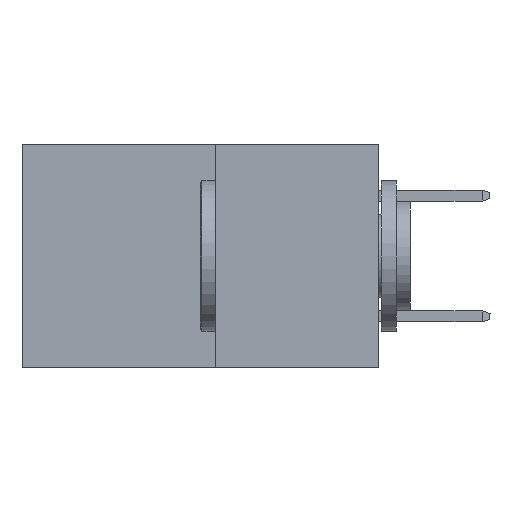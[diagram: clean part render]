
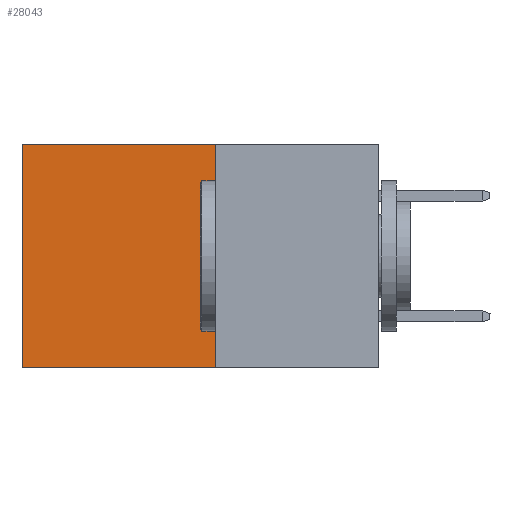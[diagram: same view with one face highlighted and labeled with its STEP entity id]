
A CAD part, left-side view. The second image highlights one B-rep face of the part: STEP entity #28043.
In plain terms, the highlighted planar face has unit normal (-1, 0, 0).
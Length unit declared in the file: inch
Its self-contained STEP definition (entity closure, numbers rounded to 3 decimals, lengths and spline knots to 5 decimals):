
#4459 = LINE ( 'NONE', #9583, #25312 ) ;
#6172 = CARTESIAN_POINT ( 'NONE',  ( 0.277, 0.27, -0.37 ) ) ;
#7576 = VERTEX_POINT ( 'NONE', #14324 ) ;
#8470 = CARTESIAN_POINT ( 'NONE',  ( 0.277, 0.27, -0.37 ) ) ;
#8761 = VECTOR ( 'NONE', #29375, 39.37008 ) ;
#8763 = LINE ( 'NONE', #15173, #21010 ) ;
#8813 = DIRECTION ( 'NONE',  ( 0., 0., -1. ) ) ;
#9583 = CARTESIAN_POINT ( 'NONE',  ( 0.277, 0.59, -0.37 ) ) ;
#9829 = CARTESIAN_POINT ( 'NONE',  ( 0.277, 0.27, 0. ) ) ;
#10429 = AXIS2_PLACEMENT_3D ( 'NONE', #6172, #24447, #8813 ) ;
#10635 = DIRECTION ( 'NONE',  ( 0., 1., 0. ) ) ;
#10711 = EDGE_CURVE ( 'NONE', #7576, #29252, #4459, .T. ) ;
#12257 = ORIENTED_EDGE ( 'NONE', *, *, #17692, .T. ) ;
#12654 = DIRECTION ( 'NONE',  ( 0., 1., 0. ) ) ;
#13452 = EDGE_LOOP ( 'NONE', ( #29640, #24329, #24765, #12257 ) ) ;
#13924 = VECTOR ( 'NONE', #10635, 39.37008 ) ;
#13949 = EDGE_CURVE ( 'NONE', #28367, #14901, #22634, .T. ) ;
#14324 = CARTESIAN_POINT ( 'NONE',  ( 0.277, 0.59, 0. ) ) ;
#14901 = VERTEX_POINT ( 'NONE', #27736 ) ;
#15173 = CARTESIAN_POINT ( 'NONE',  ( 0.277, 0.27, 0. ) ) ;
#16474 = PLANE ( 'NONE',  #10429 ) ;
#17692 = EDGE_CURVE ( 'NONE', #28367, #7576, #8763, .T. ) ;
#21010 = VECTOR ( 'NONE', #12654, 39.37008 ) ;
#22634 = LINE ( 'NONE', #8470, #8761 ) ;
#23511 = EDGE_CURVE ( 'NONE', #14901, #29252, #28611, .T. ) ;
#24329 = ORIENTED_EDGE ( 'NONE', *, *, #23511, .F. ) ;
#24447 = DIRECTION ( 'NONE',  ( 1., 0., 0. ) ) ;
#24765 = ORIENTED_EDGE ( 'NONE', *, *, #13949, .F. ) ;
#25312 = VECTOR ( 'NONE', #30484, 39.37008 ) ;
#25376 = FACE_OUTER_BOUND ( 'NONE', #13452, .T. ) ;
#27736 = CARTESIAN_POINT ( 'NONE',  ( 0.277, 0.27, -0.37 ) ) ;
#28043 = ADVANCED_FACE ( 'NONE', ( #25376 ), #16474, .F. ) ;
#28367 = VERTEX_POINT ( 'NONE', #9829 ) ;
#28611 = LINE ( 'NONE', #31402, #13924 ) ;
#29252 = VERTEX_POINT ( 'NONE', #31590 ) ;
#29375 = DIRECTION ( 'NONE',  ( 0., 0., -1. ) ) ;
#29640 = ORIENTED_EDGE ( 'NONE', *, *, #10711, .T. ) ;
#30484 = DIRECTION ( 'NONE',  ( 0., 0., -1. ) ) ;
#31402 = CARTESIAN_POINT ( 'NONE',  ( 0.277, 0.27, -0.37 ) ) ;
#31590 = CARTESIAN_POINT ( 'NONE',  ( 0.277, 0.59, -0.37 ) ) ;
